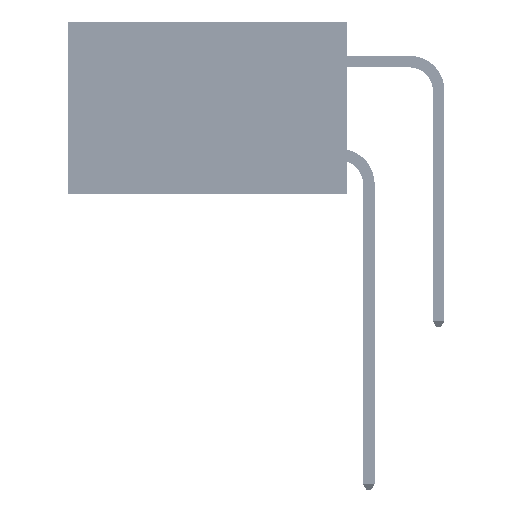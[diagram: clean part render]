
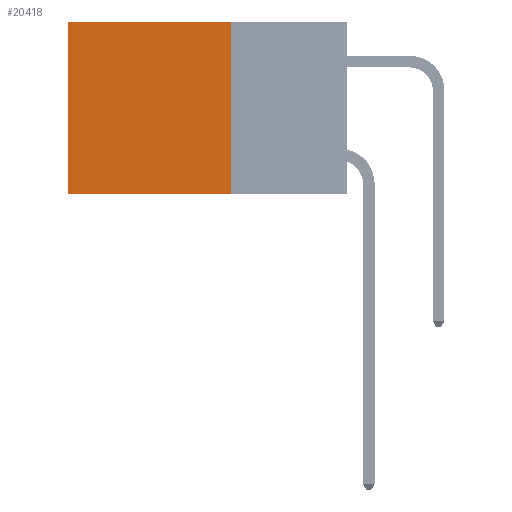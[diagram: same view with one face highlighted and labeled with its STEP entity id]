
A CAD part, left-side view. The second image highlights one B-rep face of the part: STEP entity #20418.
In plain terms, the highlighted planar face has unit normal (-1, 0, 0).
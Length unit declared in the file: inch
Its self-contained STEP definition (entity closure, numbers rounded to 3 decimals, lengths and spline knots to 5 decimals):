
#774 = ORIENTED_EDGE ( 'NONE', *, *, #25163, .F. ) ;
#3463 = LINE ( 'NONE', #4568, #20137 ) ;
#3614 = AXIS2_PLACEMENT_3D ( 'NONE', #28993, #40625, #33100 ) ;
#4568 = CARTESIAN_POINT ( 'NONE',  ( 0.2875, 0.25, -0.37 ) ) ;
#4744 = DIRECTION ( 'NONE',  ( 0., 1., 0. ) ) ;
#5240 = EDGE_LOOP ( 'NONE', ( #16349, #13207, #774, #10553 ) ) ;
#6912 = CARTESIAN_POINT ( 'NONE',  ( 0.2875, 0.25, -0.37 ) ) ;
#9668 = PLANE ( 'NONE',  #3614 ) ;
#10553 = ORIENTED_EDGE ( 'NONE', *, *, #25347, .T. ) ;
#13207 = ORIENTED_EDGE ( 'NONE', *, *, #42635, .F. ) ;
#14996 = CARTESIAN_POINT ( 'NONE',  ( 0.2875, 0.25, 0. ) ) ;
#15012 = VECTOR ( 'NONE', #47636, 39.37008 ) ;
#16349 = ORIENTED_EDGE ( 'NONE', *, *, #30286, .T. ) ;
#17160 = CARTESIAN_POINT ( 'NONE',  ( 0.2875, 0.6, 0. ) ) ;
#19128 = CARTESIAN_POINT ( 'NONE',  ( 0.2875, 0.6, 0. ) ) ;
#20137 = VECTOR ( 'NONE', #4744, 39.37008 ) ;
#20418 = ADVANCED_FACE ( 'NONE', ( #47568 ), #9668, .F. ) ;
#20624 = VERTEX_POINT ( 'NONE', #45575 ) ;
#23821 = LINE ( 'NONE', #19128, #46532 ) ;
#24264 = VERTEX_POINT ( 'NONE', #41097 ) ;
#24650 = VERTEX_POINT ( 'NONE', #17160 ) ;
#25163 = EDGE_CURVE ( 'NONE', #20624, #48149, #25543, .T. ) ;
#25347 = EDGE_CURVE ( 'NONE', #20624, #24650, #28559, .T. ) ;
#25543 = LINE ( 'NONE', #14996, #15012 ) ;
#25698 = CARTESIAN_POINT ( 'NONE',  ( 0.2875, 0.25, 0. ) ) ;
#28559 = LINE ( 'NONE', #25698, #29195 ) ;
#28993 = CARTESIAN_POINT ( 'NONE',  ( 0.2875, 0.25, 0. ) ) ;
#29195 = VECTOR ( 'NONE', #37656, 39.37008 ) ;
#30286 = EDGE_CURVE ( 'NONE', #24650, #24264, #23821, .T. ) ;
#33100 = DIRECTION ( 'NONE',  ( 0., 0., -1. ) ) ;
#37656 = DIRECTION ( 'NONE',  ( 0., 1., 0. ) ) ;
#40625 = DIRECTION ( 'NONE',  ( 1., 0., 0. ) ) ;
#41097 = CARTESIAN_POINT ( 'NONE',  ( 0.2875, 0.6, -0.37 ) ) ;
#42635 = EDGE_CURVE ( 'NONE', #48149, #24264, #3463, .T. ) ;
#45575 = CARTESIAN_POINT ( 'NONE',  ( 0.2875, 0.25, 0. ) ) ;
#46532 = VECTOR ( 'NONE', #46745, 39.37008 ) ;
#46745 = DIRECTION ( 'NONE',  ( 0., 0., -1. ) ) ;
#47568 = FACE_OUTER_BOUND ( 'NONE', #5240, .T. ) ;
#47636 = DIRECTION ( 'NONE',  ( 0., 0., -1. ) ) ;
#48149 = VERTEX_POINT ( 'NONE', #6912 ) ;
